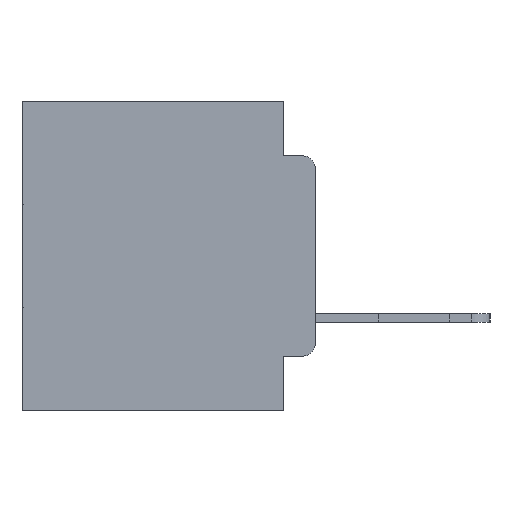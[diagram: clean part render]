
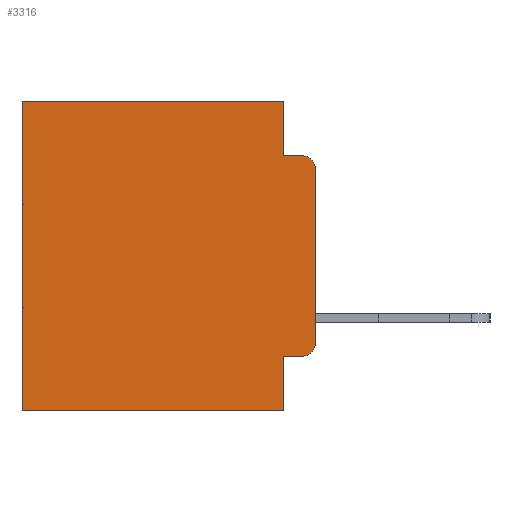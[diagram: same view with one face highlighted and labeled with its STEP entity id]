
A CAD part, left-side view. The second image highlights one B-rep face of the part: STEP entity #3316.
In plain terms, the highlighted planar face has unit normal (-1, 0, 0).
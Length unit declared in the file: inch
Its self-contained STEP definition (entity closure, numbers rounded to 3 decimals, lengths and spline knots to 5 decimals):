
#796 = VERTEX_POINT ( 'NONE', #27564 ) ;
#803 = CIRCLE ( 'NONE', #24404, 0.02 ) ;
#1382 = CARTESIAN_POINT ( 'NONE',  ( 0.298, 0.02, -0.0885 ) ) ;
#2070 = DIRECTION ( 'NONE',  ( 1., 0., 0. ) ) ;
#2076 = LINE ( 'NONE', #8378, #13877 ) ;
#2158 = CARTESIAN_POINT ( 'NONE',  ( 0.298, 0.473, -0.5 ) ) ;
#2246 = ORIENTED_EDGE ( 'NONE', *, *, #16888, .T. ) ;
#2633 = DIRECTION ( 'NONE',  ( 0., -1., 0. ) ) ;
#3028 = VERTEX_POINT ( 'NONE', #12385 ) ;
#3316 = ADVANCED_FACE ( 'NONE', ( #20892 ), #22836, .F. ) ;
#3344 = VERTEX_POINT ( 'NONE', #11779 ) ;
#3790 = EDGE_CURVE ( 'NONE', #16286, #19286, #12355, .T. ) ;
#3926 = VERTEX_POINT ( 'NONE', #29083 ) ;
#3963 = VECTOR ( 'NONE', #10126, 39.37008 ) ;
#4960 = VERTEX_POINT ( 'NONE', #16034 ) ;
#5401 = EDGE_CURVE ( 'NONE', #4960, #3926, #12976, .T. ) ;
#5423 = VECTOR ( 'NONE', #13678, 39.37008 ) ;
#6080 = CIRCLE ( 'NONE', #10705, 0.02 ) ;
#6149 = VECTOR ( 'NONE', #29567, 39.37008 ) ;
#6194 = CARTESIAN_POINT ( 'NONE',  ( 0.298, 0.473, 0. ) ) ;
#6265 = DIRECTION ( 'NONE',  ( -1., 0., 0. ) ) ;
#6357 = CARTESIAN_POINT ( 'NONE',  ( 0.298, 0., -0.1085 ) ) ;
#6546 = ORIENTED_EDGE ( 'NONE', *, *, #3790, .T. ) ;
#6768 = VECTOR ( 'NONE', #20376, 39.37008 ) ;
#8378 = CARTESIAN_POINT ( 'NONE',  ( 0.298, 0., -0.5 ) ) ;
#8931 = EDGE_LOOP ( 'NONE', ( #12582, #2246, #20778, #24365, #14980, #6546, #24604, #24770, #27616, #13616 ) ) ;
#9346 = CARTESIAN_POINT ( 'NONE',  ( 0.298, 0.02, -0.3915 ) ) ;
#9971 = CARTESIAN_POINT ( 'NONE',  ( 0.298, 0., 0. ) ) ;
#10126 = DIRECTION ( 'NONE',  ( 0., 1., 0. ) ) ;
#10215 = DIRECTION ( 'NONE',  ( 0., -1., 0. ) ) ;
#10705 = AXIS2_PLACEMENT_3D ( 'NONE', #20060, #6265, #22306 ) ;
#11627 = LINE ( 'NONE', #18205, #5423 ) ;
#11658 = EDGE_CURVE ( 'NONE', #29377, #3028, #803, .T. ) ;
#11684 = DIRECTION ( 'NONE',  ( 0., 0., -1. ) ) ;
#11779 = CARTESIAN_POINT ( 'NONE',  ( 0.298, 0.051, -0.4115 ) ) ;
#12141 = VERTEX_POINT ( 'NONE', #1382 ) ;
#12174 = DIRECTION ( 'NONE',  ( 0., 0., -1. ) ) ;
#12355 = LINE ( 'NONE', #25832, #6149 ) ;
#12385 = CARTESIAN_POINT ( 'NONE',  ( 0.298, 0., -0.3915 ) ) ;
#12582 = ORIENTED_EDGE ( 'NONE', *, *, #13798, .F. ) ;
#12976 = LINE ( 'NONE', #19544, #6768 ) ;
#13226 = EDGE_CURVE ( 'NONE', #3344, #29377, #26700, .T. ) ;
#13616 = ORIENTED_EDGE ( 'NONE', *, *, #11658, .T. ) ;
#13678 = DIRECTION ( 'NONE',  ( 0., 0., -1. ) ) ;
#13798 = EDGE_CURVE ( 'NONE', #14612, #3028, #16770, .T. ) ;
#13877 = VECTOR ( 'NONE', #28506, 39.37008 ) ;
#14298 = VECTOR ( 'NONE', #10215, 39.37008 ) ;
#14612 = VERTEX_POINT ( 'NONE', #6357 ) ;
#14693 = CARTESIAN_POINT ( 'NONE',  ( 0.298, 0., 0. ) ) ;
#14980 = ORIENTED_EDGE ( 'NONE', *, *, #24273, .T. ) ;
#16034 = CARTESIAN_POINT ( 'NONE',  ( 0.298, 0.051, 0. ) ) ;
#16286 = VERTEX_POINT ( 'NONE', #6194 ) ;
#16770 = LINE ( 'NONE', #9971, #22020 ) ;
#16888 = EDGE_CURVE ( 'NONE', #14612, #12141, #6080, .T. ) ;
#17496 = CARTESIAN_POINT ( 'NONE',  ( 0.298, 0.02, -0.4115 ) ) ;
#17859 = EDGE_CURVE ( 'NONE', #3344, #796, #11627, .T. ) ;
#18205 = CARTESIAN_POINT ( 'NONE',  ( 0.298, 0.051, 0. ) ) ;
#18536 = AXIS2_PLACEMENT_3D ( 'NONE', #26459, #2070, #12174 ) ;
#19286 = VERTEX_POINT ( 'NONE', #2158 ) ;
#19544 = CARTESIAN_POINT ( 'NONE',  ( 0.298, 0.051, 0. ) ) ;
#20060 = CARTESIAN_POINT ( 'NONE',  ( 0.298, 0.02, -0.1085 ) ) ;
#20376 = DIRECTION ( 'NONE',  ( 0., 0., -1. ) ) ;
#20778 = ORIENTED_EDGE ( 'NONE', *, *, #21369, .F. ) ;
#20892 = FACE_OUTER_BOUND ( 'NONE', #8931, .T. ) ;
#21369 = EDGE_CURVE ( 'NONE', #3926, #12141, #21387, .T. ) ;
#21387 = LINE ( 'NONE', #25493, #26411 ) ;
#21626 = LINE ( 'NONE', #14693, #3963 ) ;
#22020 = VECTOR ( 'NONE', #25668, 39.37008 ) ;
#22306 = DIRECTION ( 'NONE',  ( 0., 0., -1. ) ) ;
#22836 = PLANE ( 'NONE',  #18536 ) ;
#23576 = EDGE_CURVE ( 'NONE', #796, #19286, #2076, .T. ) ;
#23763 = CARTESIAN_POINT ( 'NONE',  ( 0.298, 0.051, -0.4115 ) ) ;
#24273 = EDGE_CURVE ( 'NONE', #4960, #16286, #21626, .T. ) ;
#24365 = ORIENTED_EDGE ( 'NONE', *, *, #5401, .F. ) ;
#24404 = AXIS2_PLACEMENT_3D ( 'NONE', #9346, #25127, #11684 ) ;
#24604 = ORIENTED_EDGE ( 'NONE', *, *, #23576, .F. ) ;
#24770 = ORIENTED_EDGE ( 'NONE', *, *, #17859, .F. ) ;
#25127 = DIRECTION ( 'NONE',  ( -1., 0., 0. ) ) ;
#25493 = CARTESIAN_POINT ( 'NONE',  ( 0.298, 0.051, -0.0885 ) ) ;
#25668 = DIRECTION ( 'NONE',  ( 0., 0., -1. ) ) ;
#25832 = CARTESIAN_POINT ( 'NONE',  ( 0.298, 0.473, 0. ) ) ;
#26411 = VECTOR ( 'NONE', #2633, 39.37008 ) ;
#26459 = CARTESIAN_POINT ( 'NONE',  ( 0.298, 0., 0. ) ) ;
#26700 = LINE ( 'NONE', #23763, #14298 ) ;
#27564 = CARTESIAN_POINT ( 'NONE',  ( 0.298, 0.051, -0.5 ) ) ;
#27616 = ORIENTED_EDGE ( 'NONE', *, *, #13226, .T. ) ;
#28506 = DIRECTION ( 'NONE',  ( 0., 1., 0. ) ) ;
#29083 = CARTESIAN_POINT ( 'NONE',  ( 0.298, 0.051, -0.0885 ) ) ;
#29377 = VERTEX_POINT ( 'NONE', #17496 ) ;
#29567 = DIRECTION ( 'NONE',  ( 0., 0., -1. ) ) ;
